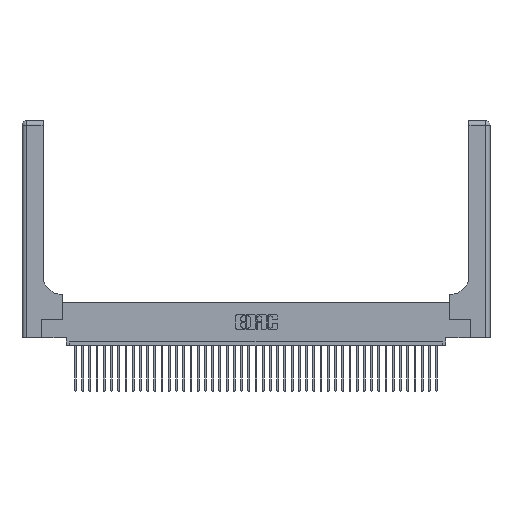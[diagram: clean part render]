
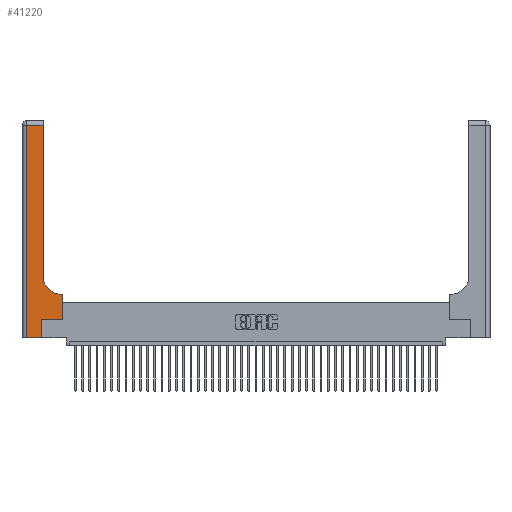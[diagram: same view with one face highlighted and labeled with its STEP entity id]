
A CAD part, top view. The second image highlights one B-rep face of the part: STEP entity #41220.
In plain terms, the highlighted planar face has unit normal (0, 0, 1).
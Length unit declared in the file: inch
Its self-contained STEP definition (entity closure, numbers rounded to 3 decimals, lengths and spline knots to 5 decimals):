
#693 = ORIENTED_EDGE ( 'NONE', *, *, #6732, .T. ) ;
#1224 = AXIS2_PLACEMENT_3D ( 'NONE', #15191, #25048, #18625 ) ;
#1468 = VERTEX_POINT ( 'NONE', #7201 ) ;
#1607 = CARTESIAN_POINT ( 'NONE',  ( 0.2915, 3., 0.37 ) ) ;
#2177 = PLANE ( 'NONE',  #32098 ) ;
#2914 = DIRECTION ( 'NONE',  ( 0., -1., 0. ) ) ;
#4441 = CIRCLE ( 'NONE', #1224, 0.25 ) ;
#5010 = CARTESIAN_POINT ( 'NONE',  ( 0.06, 0., 0.37 ) ) ;
#6732 = EDGE_CURVE ( 'NONE', #33720, #33868, #12951, .T. ) ;
#7201 = CARTESIAN_POINT ( 'NONE',  ( 0.06, 2.94, 0.37 ) ) ;
#8652 = ORIENTED_EDGE ( 'NONE', *, *, #25638, .T. ) ;
#8690 = CARTESIAN_POINT ( 'NONE',  ( 0.269, 0., 0.37 ) ) ;
#8777 = CARTESIAN_POINT ( 'NONE',  ( 0.2915, 2.94, 0.37 ) ) ;
#8880 = CARTESIAN_POINT ( 'NONE',  ( 0.5585, 0.25, 0.37 ) ) ;
#11365 = ORIENTED_EDGE ( 'NONE', *, *, #15414, .T. ) ;
#11768 = CARTESIAN_POINT ( 'NONE',  ( 0., 2.94, 0.37 ) ) ;
#12951 = LINE ( 'NONE', #25545, #42199 ) ;
#12973 = LINE ( 'NONE', #32548, #38611 ) ;
#15191 = CARTESIAN_POINT ( 'NONE',  ( 0.5415, 0.85, 0.37 ) ) ;
#15414 = EDGE_CURVE ( 'NONE', #32281, #31294, #4441, .T. ) ;
#15517 = VECTOR ( 'NONE', #42406, 39.37008 ) ;
#15937 = CARTESIAN_POINT ( 'NONE',  ( 0.5415, 0.6, 0.37 ) ) ;
#16097 = DIRECTION ( 'NONE',  ( 1., 0., 0. ) ) ;
#18495 = EDGE_CURVE ( 'NONE', #40574, #33720, #36272, .T. ) ;
#18625 = DIRECTION ( 'NONE',  ( 1., 0., 0. ) ) ;
#18706 = ORIENTED_EDGE ( 'NONE', *, *, #26962, .T. ) ;
#18925 = CARTESIAN_POINT ( 'NONE',  ( 0.5585, 0.6, 0.37 ) ) ;
#20060 = VECTOR ( 'NONE', #16097, 39.37008 ) ;
#20461 = DIRECTION ( 'NONE',  ( 0., 1., 0. ) ) ;
#21250 = EDGE_CURVE ( 'NONE', #1468, #21558, #22680, .T. ) ;
#21558 = VERTEX_POINT ( 'NONE', #5010 ) ;
#22680 = LINE ( 'NONE', #38649, #33986 ) ;
#22992 = ORIENTED_EDGE ( 'NONE', *, *, #26203, .T. ) ;
#23173 = EDGE_LOOP ( 'NONE', ( #38707, #38000, #37276, #18706, #42368, #693, #8652, #22992, #11365 ) ) ;
#23189 = DIRECTION ( 'NONE',  ( 0., 1., 0. ) ) ;
#25048 = DIRECTION ( 'NONE',  ( 0., 0., -1. ) ) ;
#25545 = CARTESIAN_POINT ( 'NONE',  ( 0.269, 0.25, 0.37 ) ) ;
#25638 = EDGE_CURVE ( 'NONE', #33868, #38847, #12973, .T. ) ;
#25692 = CARTESIAN_POINT ( 'NONE',  ( 0., 0., 0.37 ) ) ;
#26035 = CARTESIAN_POINT ( 'NONE',  ( 0.2915, 0.6, 0.37 ) ) ;
#26203 = EDGE_CURVE ( 'NONE', #38847, #32281, #39652, .T. ) ;
#26962 = EDGE_CURVE ( 'NONE', #21558, #40574, #28801, .T. ) ;
#27360 = CARTESIAN_POINT ( 'NONE',  ( 0.269, 0.25, 0.37 ) ) ;
#27520 = VECTOR ( 'NONE', #20461, 39.37008 ) ;
#28406 = DIRECTION ( 'NONE',  ( -1., 0., 0. ) ) ;
#28801 = LINE ( 'NONE', #25692, #20060 ) ;
#29715 = VERTEX_POINT ( 'NONE', #8777 ) ;
#31127 = VECTOR ( 'NONE', #41197, 39.37008 ) ;
#31294 = VERTEX_POINT ( 'NONE', #34059 ) ;
#31441 = DIRECTION ( 'NONE',  ( 0., 0., -1. ) ) ;
#31554 = DIRECTION ( 'NONE',  ( -1., 0., 0. ) ) ;
#32098 = AXIS2_PLACEMENT_3D ( 'NONE', #41475, #31441, #28406 ) ;
#32274 = LINE ( 'NONE', #11768, #32624 ) ;
#32281 = VERTEX_POINT ( 'NONE', #15937 ) ;
#32548 = CARTESIAN_POINT ( 'NONE',  ( 0.5585, 0.25, 0.37 ) ) ;
#32624 = VECTOR ( 'NONE', #31554, 39.37008 ) ;
#33720 = VERTEX_POINT ( 'NONE', #27360 ) ;
#33868 = VERTEX_POINT ( 'NONE', #8880 ) ;
#33986 = VECTOR ( 'NONE', #2914, 39.37008 ) ;
#34059 = CARTESIAN_POINT ( 'NONE',  ( 0.2915, 0.85, 0.37 ) ) ;
#34086 = FACE_OUTER_BOUND ( 'NONE', #23173, .T. ) ;
#35450 = DIRECTION ( 'NONE',  ( 1., 0., 0. ) ) ;
#36035 = EDGE_CURVE ( 'NONE', #31294, #29715, #37811, .T. ) ;
#36272 = LINE ( 'NONE', #40144, #27520 ) ;
#37276 = ORIENTED_EDGE ( 'NONE', *, *, #21250, .T. ) ;
#37811 = LINE ( 'NONE', #1607, #31127 ) ;
#38000 = ORIENTED_EDGE ( 'NONE', *, *, #38745, .T. ) ;
#38611 = VECTOR ( 'NONE', #23189, 39.37008 ) ;
#38649 = CARTESIAN_POINT ( 'NONE',  ( 0.06, 3., 0.37 ) ) ;
#38707 = ORIENTED_EDGE ( 'NONE', *, *, #36035, .T. ) ;
#38745 = EDGE_CURVE ( 'NONE', #29715, #1468, #32274, .T. ) ;
#38847 = VERTEX_POINT ( 'NONE', #18925 ) ;
#39652 = LINE ( 'NONE', #26035, #15517 ) ;
#40144 = CARTESIAN_POINT ( 'NONE',  ( 0.269, 0., 0.37 ) ) ;
#40574 = VERTEX_POINT ( 'NONE', #8690 ) ;
#41197 = DIRECTION ( 'NONE',  ( 0., 1., 0. ) ) ;
#41220 = ADVANCED_FACE ( 'NONE', ( #34086 ), #2177, .F. ) ;
#41475 = CARTESIAN_POINT ( 'NONE',  ( 0., 3., 0.37 ) ) ;
#42199 = VECTOR ( 'NONE', #35450, 39.37008 ) ;
#42368 = ORIENTED_EDGE ( 'NONE', *, *, #18495, .T. ) ;
#42406 = DIRECTION ( 'NONE',  ( -1., 0., 0. ) ) ;
